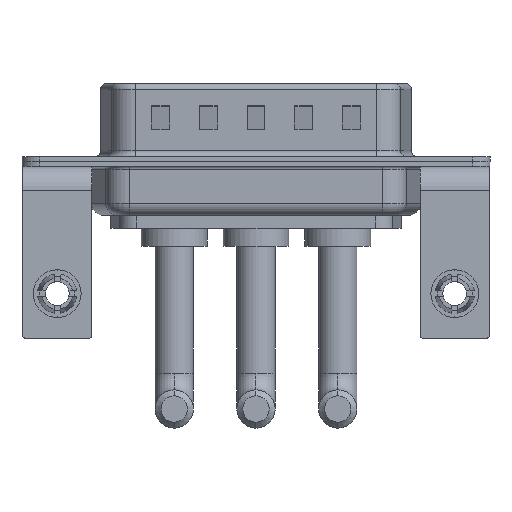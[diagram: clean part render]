
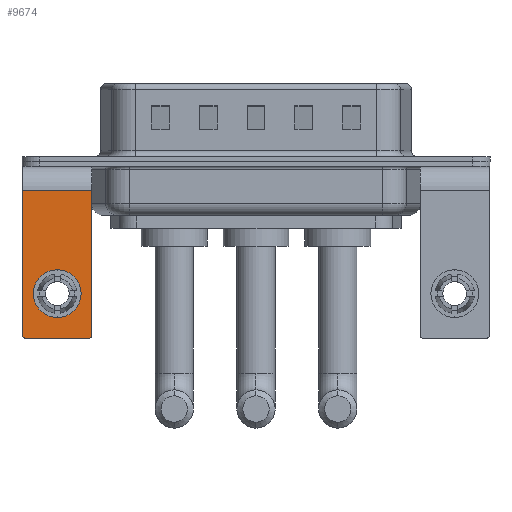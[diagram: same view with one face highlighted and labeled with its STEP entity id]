
A CAD part, front view. The second image highlights one B-rep face of the part: STEP entity #9674.
In plain terms, the highlighted planar face has unit normal (0, -1, 0).
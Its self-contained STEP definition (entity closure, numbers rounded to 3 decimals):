
#95 = DIRECTION ( 'NONE',  ( 0., 0., 1. ) ) ;
#1161 = FACE_BOUND ( 'NONE', #9719, .T. ) ;
#1531 = CARTESIAN_POINT ( 'NONE',  ( 2.65, -6.25, -14.55 ) ) ;
#1577 = CARTESIAN_POINT ( 'NONE',  ( 2.9, -6.25, -14.8 ) ) ;
#1646 = VECTOR ( 'NONE', #14516, 1000. ) ;
#1924 = AXIS2_PLACEMENT_3D ( 'NONE', #2012, #12889, #7582 ) ;
#2012 = CARTESIAN_POINT ( 'NONE',  ( 0., -6.25, -11.07 ) ) ;
#2163 = CARTESIAN_POINT ( 'NONE',  ( -2.65, -6.25, -14.8 ) ) ;
#2187 = DIRECTION ( 'NONE',  ( 0., 0., 1. ) ) ;
#2309 = EDGE_CURVE ( 'NONE', #17174, #8189, #14069, .T. ) ;
#2826 = EDGE_CURVE ( 'NONE', #9442, #7790, #14676, .T. ) ;
#3328 = LINE ( 'NONE', #8826, #7591 ) ;
#3401 = CARTESIAN_POINT ( 'NONE',  ( -2.9, -6.25, -14.55 ) ) ;
#3444 = EDGE_CURVE ( 'NONE', #9442, #14278, #3328, .T. ) ;
#4532 = ORIENTED_EDGE ( 'NONE', *, *, #5859, .T. ) ;
#4927 = AXIS2_PLACEMENT_3D ( 'NONE', #1531, #15756, #14284 ) ;
#5117 = DIRECTION ( 'NONE',  ( 0., 1., 0. ) ) ;
#5850 = CARTESIAN_POINT ( 'NONE',  ( -2.9, -6.25, -2.4 ) ) ;
#5859 = EDGE_CURVE ( 'NONE', #14278, #10255, #6220, .T. ) ;
#5872 = EDGE_CURVE ( 'NONE', #12984, #13883, #7771, .T. ) ;
#6174 = ORIENTED_EDGE ( 'NONE', *, *, #3444, .T. ) ;
#6220 = LINE ( 'NONE', #14431, #1646 ) ;
#6364 = AXIS2_PLACEMENT_3D ( 'NONE', #12616, #14058, #95 ) ;
#6387 = CARTESIAN_POINT ( 'NONE',  ( 0., -6.25, -11.07 ) ) ;
#6471 = CARTESIAN_POINT ( 'NONE',  ( 2.9, -6.25, -14.55 ) ) ;
#6738 = CARTESIAN_POINT ( 'NONE',  ( 2.9, -6.25, -2.4 ) ) ;
#6921 = ORIENTED_EDGE ( 'NONE', *, *, #7545, .T. ) ;
#7125 = VECTOR ( 'NONE', #7143, 1000. ) ;
#7143 = DIRECTION ( 'NONE',  ( -1., 0., 0. ) ) ;
#7545 = EDGE_CURVE ( 'NONE', #10255, #8189, #8122, .T. ) ;
#7582 = DIRECTION ( 'NONE',  ( 0., 0., 1. ) ) ;
#7591 = VECTOR ( 'NONE', #14385, 1000. ) ;
#7771 = CIRCLE ( 'NONE', #1924, 2. ) ;
#7790 = VERTEX_POINT ( 'NONE', #6471 ) ;
#8122 = CIRCLE ( 'NONE', #6364, 0.25 ) ;
#8189 = VERTEX_POINT ( 'NONE', #2163 ) ;
#8448 = CARTESIAN_POINT ( 'NONE',  ( 0., -6.25, -9.07 ) ) ;
#8527 = EDGE_LOOP ( 'NONE', ( #4532, #6921, #13073, #11008, #16249, #6174 ) ) ;
#8750 = AXIS2_PLACEMENT_3D ( 'NONE', #6387, #5117, #2187 ) ;
#8751 = CARTESIAN_POINT ( 'NONE',  ( 2.9, -6.25, -2.4 ) ) ;
#8826 = CARTESIAN_POINT ( 'NONE',  ( 2.9, -6.25, -2.4 ) ) ;
#9283 = FACE_OUTER_BOUND ( 'NONE', #8527, .T. ) ;
#9285 = AXIS2_PLACEMENT_3D ( 'NONE', #6738, #13378, #16327 ) ;
#9442 = VERTEX_POINT ( 'NONE', #11753 ) ;
#9674 = ADVANCED_FACE ( 'NONE', ( #1161, #9283 ), #12114, .F. ) ;
#9719 = EDGE_LOOP ( 'NONE', ( #17980, #17782 ) ) ;
#10033 = EDGE_CURVE ( 'NONE', #17174, #7790, #13358, .T. ) ;
#10035 = CARTESIAN_POINT ( 'NONE',  ( 2.65, -6.25, -14.8 ) ) ;
#10255 = VERTEX_POINT ( 'NONE', #3401 ) ;
#10779 = EDGE_CURVE ( 'NONE', #13883, #12984, #13985, .T. ) ;
#11008 = ORIENTED_EDGE ( 'NONE', *, *, #10033, .T. ) ;
#11753 = CARTESIAN_POINT ( 'NONE',  ( 2.9, -6.25, -2.4 ) ) ;
#12114 = PLANE ( 'NONE',  #9285 ) ;
#12616 = CARTESIAN_POINT ( 'NONE',  ( -2.65, -6.25, -14.55 ) ) ;
#12699 = VECTOR ( 'NONE', #15688, 1000. ) ;
#12889 = DIRECTION ( 'NONE',  ( 0., 1., 0. ) ) ;
#12984 = VERTEX_POINT ( 'NONE', #8448 ) ;
#13073 = ORIENTED_EDGE ( 'NONE', *, *, #2309, .F. ) ;
#13318 = CARTESIAN_POINT ( 'NONE',  ( 0., -6.25, -13.07 ) ) ;
#13358 = CIRCLE ( 'NONE', #4927, 0.25 ) ;
#13378 = DIRECTION ( 'NONE',  ( 0., 1., 0. ) ) ;
#13883 = VERTEX_POINT ( 'NONE', #13318 ) ;
#13985 = CIRCLE ( 'NONE', #8750, 2. ) ;
#14058 = DIRECTION ( 'NONE',  ( 0., -1., 0. ) ) ;
#14069 = LINE ( 'NONE', #1577, #7125 ) ;
#14278 = VERTEX_POINT ( 'NONE', #5850 ) ;
#14284 = DIRECTION ( 'NONE',  ( 0., 0., 1. ) ) ;
#14385 = DIRECTION ( 'NONE',  ( -1., 0., 0. ) ) ;
#14431 = CARTESIAN_POINT ( 'NONE',  ( -2.9, -6.25, -2.4 ) ) ;
#14516 = DIRECTION ( 'NONE',  ( 0., 0., -1. ) ) ;
#14676 = LINE ( 'NONE', #8751, #12699 ) ;
#15688 = DIRECTION ( 'NONE',  ( 0., 0., -1. ) ) ;
#15756 = DIRECTION ( 'NONE',  ( 0., -1., 0. ) ) ;
#16249 = ORIENTED_EDGE ( 'NONE', *, *, #2826, .F. ) ;
#16327 = DIRECTION ( 'NONE',  ( 0., 0., 1. ) ) ;
#17174 = VERTEX_POINT ( 'NONE', #10035 ) ;
#17782 = ORIENTED_EDGE ( 'NONE', *, *, #5872, .T. ) ;
#17980 = ORIENTED_EDGE ( 'NONE', *, *, #10779, .T. ) ;
